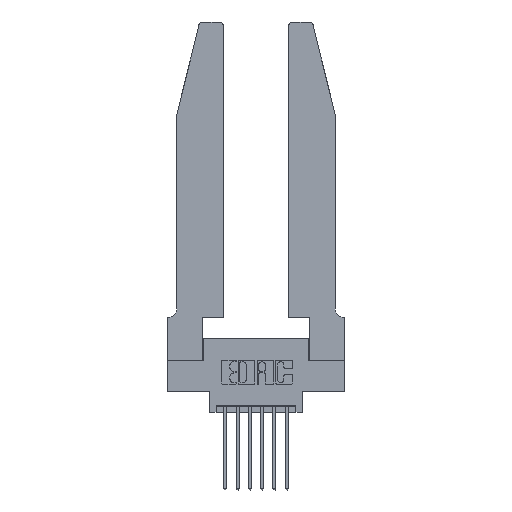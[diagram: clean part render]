
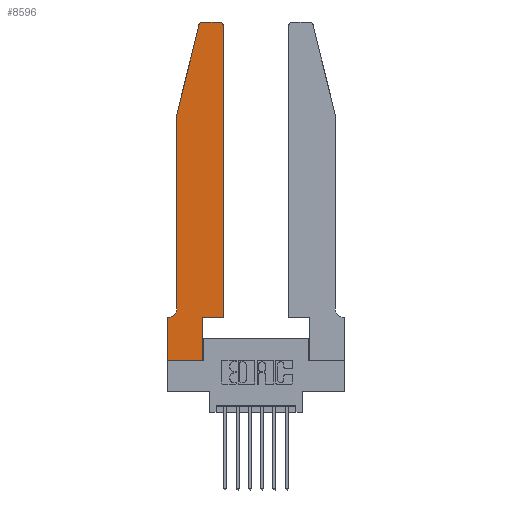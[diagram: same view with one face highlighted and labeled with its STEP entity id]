
A CAD part, top view. The second image highlights one B-rep face of the part: STEP entity #8596.
In plain terms, the highlighted planar face has unit normal (0, 0, 1).
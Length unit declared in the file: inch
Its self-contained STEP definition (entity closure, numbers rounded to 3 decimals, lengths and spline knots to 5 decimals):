
#217 = ORIENTED_EDGE ( 'NONE', *, *, #13919, .T. ) ;
#365 = VERTEX_POINT ( 'NONE', #14425 ) ;
#690 = DIRECTION ( 'NONE',  ( 1., 0., 0. ) ) ;
#872 = CARTESIAN_POINT ( 'NONE',  ( 0., 0.35, 0.37 ) ) ;
#1067 = EDGE_CURVE ( 'NONE', #2889, #3595, #9241, .T. ) ;
#1128 = CARTESIAN_POINT ( 'NONE',  ( 0., 0., 0.37 ) ) ;
#1209 = AXIS2_PLACEMENT_3D ( 'NONE', #9300, #2630, #10436 ) ;
#1326 = VECTOR ( 'NONE', #8389, 39.37008 ) ;
#1391 = DIRECTION ( 'NONE',  ( 0., 1., 0. ) ) ;
#1412 = VERTEX_POINT ( 'NONE', #4720 ) ;
#1590 = LINE ( 'NONE', #4901, #13078 ) ;
#1733 = CARTESIAN_POINT ( 'NONE',  ( 0.4505, 2.72, 0.37 ) ) ;
#1748 = CIRCLE ( 'NONE', #10943, 0.03 ) ;
#2085 = ORIENTED_EDGE ( 'NONE', *, *, #5455, .T. ) ;
#2231 = DIRECTION ( 'NONE',  ( 1., 0., 0. ) ) ;
#2265 = VECTOR ( 'NONE', #11905, 39.37008 ) ;
#2630 = DIRECTION ( 'NONE',  ( 0., 0., 1. ) ) ;
#2789 = VECTOR ( 'NONE', #4274, 39.37008 ) ;
#2889 = VERTEX_POINT ( 'NONE', #12008 ) ;
#3033 = CARTESIAN_POINT ( 'NONE',  ( 0.0055, 0.42, 0.37 ) ) ;
#3052 = EDGE_CURVE ( 'NONE', #11068, #8158, #1590, .T. ) ;
#3074 = CARTESIAN_POINT ( 'NONE',  ( 0.2865, 0.35, 0.37 ) ) ;
#3152 = CARTESIAN_POINT ( 'NONE',  ( 0., 0., 0.37 ) ) ;
#3307 = VECTOR ( 'NONE', #12627, 39.37008 ) ;
#3425 = VERTEX_POINT ( 'NONE', #11409 ) ;
#3460 = VECTOR ( 'NONE', #1391, 39.37008 ) ;
#3521 = VERTEX_POINT ( 'NONE', #10624 ) ;
#3595 = VERTEX_POINT ( 'NONE', #11448 ) ;
#3832 = ORIENTED_EDGE ( 'NONE', *, *, #14374, .T. ) ;
#3867 = VERTEX_POINT ( 'NONE', #5511 ) ;
#4040 = ORIENTED_EDGE ( 'NONE', *, *, #4785, .T. ) ;
#4065 = VECTOR ( 'NONE', #4747, 39.37008 ) ;
#4151 = DIRECTION ( 'NONE',  ( -1., 0., 0. ) ) ;
#4274 = DIRECTION ( 'NONE',  ( 0., -1., 0. ) ) ;
#4430 = FACE_OUTER_BOUND ( 'NONE', #11291, .T. ) ;
#4478 = CARTESIAN_POINT ( 'NONE',  ( 0., 0.35, 0.37 ) ) ;
#4525 = EDGE_CURVE ( 'NONE', #6041, #365, #1748, .T. ) ;
#4606 = VECTOR ( 'NONE', #690, 39.37008 ) ;
#4650 = CARTESIAN_POINT ( 'NONE',  ( 0.0755, 2., 0.37 ) ) ;
#4720 = CARTESIAN_POINT ( 'NONE',  ( 0.25487, 2.72718, 0.37 ) ) ;
#4747 = DIRECTION ( 'NONE',  ( -0.239, -0.971, 0. ) ) ;
#4785 = EDGE_CURVE ( 'NONE', #3425, #9463, #10478, .T. ) ;
#4901 = CARTESIAN_POINT ( 'NONE',  ( 0.0755, 2., 0.37 ) ) ;
#5324 = ORIENTED_EDGE ( 'NONE', *, *, #8858, .T. ) ;
#5330 = DIRECTION ( 'NONE',  ( 0., -1., 0. ) ) ;
#5455 = EDGE_CURVE ( 'NONE', #8158, #3425, #7670, .T. ) ;
#5511 = CARTESIAN_POINT ( 'NONE',  ( 0.284, 2.75, 0.37 ) ) ;
#5837 = EDGE_CURVE ( 'NONE', #11562, #6041, #12688, .T. ) ;
#5844 = ORIENTED_EDGE ( 'NONE', *, *, #11589, .T. ) ;
#5845 = CARTESIAN_POINT ( 'NONE',  ( 0.4505, 0.35, 0.37 ) ) ;
#6041 = VERTEX_POINT ( 'NONE', #1733 ) ;
#6371 = AXIS2_PLACEMENT_3D ( 'NONE', #3033, #10834, #4151 ) ;
#6493 = ORIENTED_EDGE ( 'NONE', *, *, #10894, .T. ) ;
#6533 = ORIENTED_EDGE ( 'NONE', *, *, #4525, .T. ) ;
#6621 = CARTESIAN_POINT ( 'NONE',  ( 0.0755, 2., 0.37 ) ) ;
#6724 = PLANE ( 'NONE',  #8264 ) ;
#7001 = CARTESIAN_POINT ( 'NONE',  ( 0.0755, 0.42, 0.37 ) ) ;
#7307 = LINE ( 'NONE', #11737, #1326 ) ;
#7586 = LINE ( 'NONE', #14027, #4606 ) ;
#7670 = CIRCLE ( 'NONE', #6371, 0.07 ) ;
#7741 = CARTESIAN_POINT ( 'NONE',  ( 0.0755, 0.35, 0.37 ) ) ;
#7846 = DIRECTION ( 'NONE',  ( 1., 0., 0. ) ) ;
#7870 = LINE ( 'NONE', #3074, #2265 ) ;
#8158 = VERTEX_POINT ( 'NONE', #7001 ) ;
#8264 = AXIS2_PLACEMENT_3D ( 'NONE', #4478, #14471, #7846 ) ;
#8389 = DIRECTION ( 'NONE',  ( -1., 0., 0. ) ) ;
#8596 = ADVANCED_FACE ( 'NONE', ( #4430 ), #6724, .T. ) ;
#8858 = EDGE_CURVE ( 'NONE', #3521, #11562, #7586, .T. ) ;
#9241 = LINE ( 'NONE', #1128, #3307 ) ;
#9300 = CARTESIAN_POINT ( 'NONE',  ( 0.284, 2.72, 0.37 ) ) ;
#9463 = VERTEX_POINT ( 'NONE', #872 ) ;
#9721 = EDGE_CURVE ( 'NONE', #1412, #11068, #12584, .T. ) ;
#9754 = DIRECTION ( 'NONE',  ( 0., 0., 1. ) ) ;
#9771 = CARTESIAN_POINT ( 'NONE',  ( 0.4505, 0.35, 0.37 ) ) ;
#9772 = CARTESIAN_POINT ( 'NONE',  ( 0.4205, 2.72, 0.37 ) ) ;
#9853 = ORIENTED_EDGE ( 'NONE', *, *, #5837, .T. ) ;
#9958 = DIRECTION ( 'NONE',  ( -1., 0., 0. ) ) ;
#10436 = DIRECTION ( 'NONE',  ( 1., 0., 0. ) ) ;
#10478 = LINE ( 'NONE', #7741, #13417 ) ;
#10624 = CARTESIAN_POINT ( 'NONE',  ( 0.2865, 0.35, 0.37 ) ) ;
#10834 = DIRECTION ( 'NONE',  ( 0., 0., -1. ) ) ;
#10894 = EDGE_CURVE ( 'NONE', #3595, #3521, #7870, .T. ) ;
#10943 = AXIS2_PLACEMENT_3D ( 'NONE', #9772, #9754, #2231 ) ;
#11068 = VERTEX_POINT ( 'NONE', #6621 ) ;
#11291 = EDGE_LOOP ( 'NONE', ( #217, #3832, #13198, #13960, #2085, #4040, #5844, #12089, #6493, #5324, #9853, #6533 ) ) ;
#11409 = CARTESIAN_POINT ( 'NONE',  ( 0.0055, 0.35, 0.37 ) ) ;
#11448 = CARTESIAN_POINT ( 'NONE',  ( 0.2865, 0., 0.37 ) ) ;
#11562 = VERTEX_POINT ( 'NONE', #9771 ) ;
#11589 = EDGE_CURVE ( 'NONE', #9463, #2889, #14243, .T. ) ;
#11737 = CARTESIAN_POINT ( 'NONE',  ( 0.2605, 2.75, 0.37 ) ) ;
#11905 = DIRECTION ( 'NONE',  ( 0., 1., 0. ) ) ;
#12008 = CARTESIAN_POINT ( 'NONE',  ( 0., 0., 0.37 ) ) ;
#12089 = ORIENTED_EDGE ( 'NONE', *, *, #1067, .T. ) ;
#12584 = LINE ( 'NONE', #4650, #4065 ) ;
#12627 = DIRECTION ( 'NONE',  ( 1., 0., 0. ) ) ;
#12688 = LINE ( 'NONE', #5845, #3460 ) ;
#13078 = VECTOR ( 'NONE', #5330, 39.37008 ) ;
#13198 = ORIENTED_EDGE ( 'NONE', *, *, #9721, .T. ) ;
#13417 = VECTOR ( 'NONE', #9958, 39.37008 ) ;
#13516 = CIRCLE ( 'NONE', #1209, 0.03 ) ;
#13919 = EDGE_CURVE ( 'NONE', #365, #3867, #7307, .T. ) ;
#13960 = ORIENTED_EDGE ( 'NONE', *, *, #3052, .T. ) ;
#14027 = CARTESIAN_POINT ( 'NONE',  ( 0.4505, 0.35, 0.37 ) ) ;
#14243 = LINE ( 'NONE', #3152, #2789 ) ;
#14374 = EDGE_CURVE ( 'NONE', #3867, #1412, #13516, .T. ) ;
#14425 = CARTESIAN_POINT ( 'NONE',  ( 0.4205, 2.75, 0.37 ) ) ;
#14471 = DIRECTION ( 'NONE',  ( 0., 0., 1. ) ) ;
